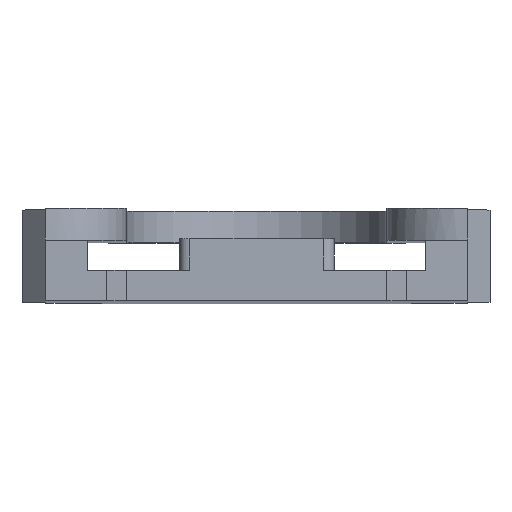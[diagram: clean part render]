
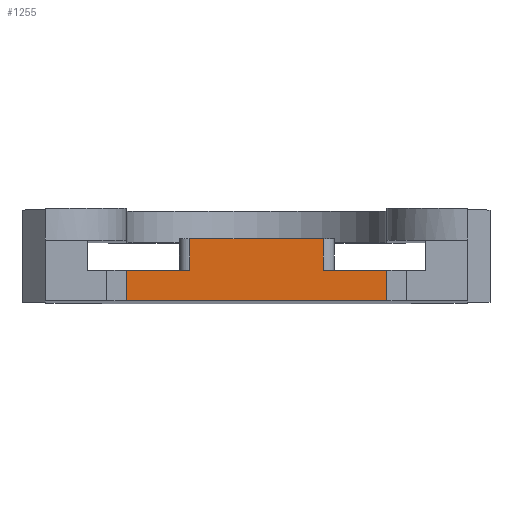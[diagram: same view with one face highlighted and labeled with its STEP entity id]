
A CAD part, top view. The second image highlights one B-rep face of the part: STEP entity #1255.
In plain terms, the highlighted planar face has unit normal (0, 0, 1).
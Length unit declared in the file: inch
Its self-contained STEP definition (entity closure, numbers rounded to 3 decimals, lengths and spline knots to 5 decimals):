
#4 = VECTOR ( 'NONE', #243, 39.37008 ) ;
#11 = EDGE_CURVE ( 'NONE', #1223, #1019, #655, .T. ) ;
#63 = LINE ( 'NONE', #1146, #574 ) ;
#65 = VECTOR ( 'NONE', #263, 39.37008 ) ;
#67 = EDGE_LOOP ( 'NONE', ( #666, #165, #1251, #322, #742, #814, #377, #841 ) ) ;
#124 = VECTOR ( 'NONE', #691, 39.37008 ) ;
#125 = CARTESIAN_POINT ( 'NONE',  ( -0.205, 0.088, 0. ) ) ;
#150 = CARTESIAN_POINT ( 'NONE',  ( -0.395, 0.088, 0. ) ) ;
#165 = ORIENTED_EDGE ( 'NONE', *, *, #768, .F. ) ;
#190 = LINE ( 'NONE', #879, #1052 ) ;
#243 = DIRECTION ( 'NONE',  ( 0., -1., 0. ) ) ;
#263 = DIRECTION ( 'NONE',  ( 0., -1., 0. ) ) ;
#271 = LINE ( 'NONE', #645, #4 ) ;
#293 = CARTESIAN_POINT ( 'NONE',  ( 0., 0.131, 0. ) ) ;
#304 = VECTOR ( 'NONE', #854, 39.37008 ) ;
#322 = ORIENTED_EDGE ( 'NONE', *, *, #956, .F. ) ;
#338 = LINE ( 'NONE', #1142, #65 ) ;
#363 = CARTESIAN_POINT ( 'NONE',  ( -0.115, 0., 0. ) ) ;
#377 = ORIENTED_EDGE ( 'NONE', *, *, #1133, .T. ) ;
#438 = VERTEX_POINT ( 'NONE', #1087 ) ;
#448 = CARTESIAN_POINT ( 'NONE',  ( -0.115, 0.045, 0. ) ) ;
#491 = EDGE_CURVE ( 'NONE', #934, #438, #338, .T. ) ;
#497 = CARTESIAN_POINT ( 'NONE',  ( -0.485, 0., 0. ) ) ;
#503 = DIRECTION ( 'NONE',  ( 0., 0., 1. ) ) ;
#510 = DIRECTION ( 'NONE',  ( 0., -1., 0. ) ) ;
#532 = VECTOR ( 'NONE', #1024, 39.37008 ) ;
#574 = VECTOR ( 'NONE', #1046, 39.37008 ) ;
#583 = VERTEX_POINT ( 'NONE', #497 ) ;
#584 = AXIS2_PLACEMENT_3D ( 'NONE', #293, #503, #1197 ) ;
#645 = CARTESIAN_POINT ( 'NONE',  ( -0.205, 0.088, 0. ) ) ;
#655 = LINE ( 'NONE', #448, #716 ) ;
#666 = ORIENTED_EDGE ( 'NONE', *, *, #11, .F. ) ;
#691 = DIRECTION ( 'NONE',  ( 1., 0., 0. ) ) ;
#697 = VERTEX_POINT ( 'NONE', #713 ) ;
#713 = CARTESIAN_POINT ( 'NONE',  ( -0.205, 0.043, 0. ) ) ;
#716 = VECTOR ( 'NONE', #510, 39.37008 ) ;
#725 = CARTESIAN_POINT ( 'NONE',  ( -0.54, 0.043, 0. ) ) ;
#742 = ORIENTED_EDGE ( 'NONE', *, *, #491, .T. ) ;
#747 = FACE_OUTER_BOUND ( 'NONE', #67, .T. ) ;
#754 = LINE ( 'NONE', #725, #532 ) ;
#768 = EDGE_CURVE ( 'NONE', #697, #1223, #754, .T. ) ;
#773 = LINE ( 'NONE', #150, #304 ) ;
#793 = PLANE ( 'NONE',  #584 ) ;
#811 = VERTEX_POINT ( 'NONE', #125 ) ;
#814 = ORIENTED_EDGE ( 'NONE', *, *, #1232, .F. ) ;
#841 = ORIENTED_EDGE ( 'NONE', *, *, #913, .F. ) ;
#854 = DIRECTION ( 'NONE',  ( 1., 0., 0. ) ) ;
#879 = CARTESIAN_POINT ( 'NONE',  ( -0.485, 0.045, 0. ) ) ;
#913 = EDGE_CURVE ( 'NONE', #1019, #583, #63, .T. ) ;
#934 = VERTEX_POINT ( 'NONE', #943 ) ;
#943 = CARTESIAN_POINT ( 'NONE',  ( -0.395, 0.088, 0. ) ) ;
#951 = EDGE_CURVE ( 'NONE', #811, #697, #271, .T. ) ;
#956 = EDGE_CURVE ( 'NONE', #934, #811, #773, .T. ) ;
#1019 = VERTEX_POINT ( 'NONE', #363 ) ;
#1024 = DIRECTION ( 'NONE',  ( 1., 0., 0. ) ) ;
#1046 = DIRECTION ( 'NONE',  ( -1., 0., 0. ) ) ;
#1052 = VECTOR ( 'NONE', #1278, 39.37008 ) ;
#1084 = LINE ( 'NONE', #1096, #124 ) ;
#1087 = CARTESIAN_POINT ( 'NONE',  ( -0.395, 0.043, 0. ) ) ;
#1096 = CARTESIAN_POINT ( 'NONE',  ( -0.54, 0.043, 0. ) ) ;
#1105 = CARTESIAN_POINT ( 'NONE',  ( -0.485, 0.043, 0. ) ) ;
#1133 = EDGE_CURVE ( 'NONE', #1271, #583, #190, .T. ) ;
#1142 = CARTESIAN_POINT ( 'NONE',  ( -0.395, 0.088, 0. ) ) ;
#1146 = CARTESIAN_POINT ( 'NONE',  ( 0., 0., 0. ) ) ;
#1190 = CARTESIAN_POINT ( 'NONE',  ( -0.115, 0.043, 0. ) ) ;
#1197 = DIRECTION ( 'NONE',  ( 1., 0., 0. ) ) ;
#1223 = VERTEX_POINT ( 'NONE', #1190 ) ;
#1232 = EDGE_CURVE ( 'NONE', #1271, #438, #1084, .T. ) ;
#1251 = ORIENTED_EDGE ( 'NONE', *, *, #951, .F. ) ;
#1255 = ADVANCED_FACE ( 'NONE', ( #747 ), #793, .T. ) ;
#1271 = VERTEX_POINT ( 'NONE', #1105 ) ;
#1278 = DIRECTION ( 'NONE',  ( 0., -1., 0. ) ) ;
